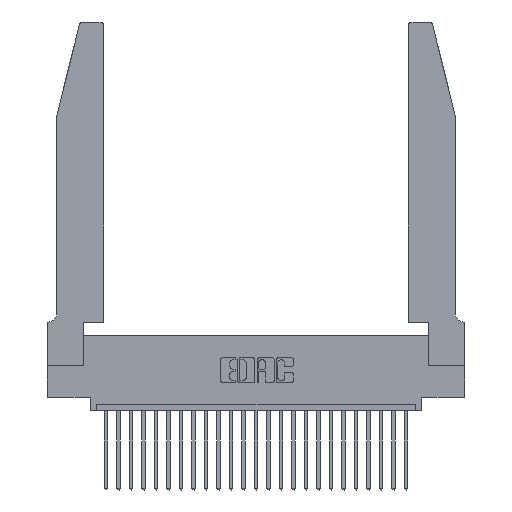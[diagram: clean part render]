
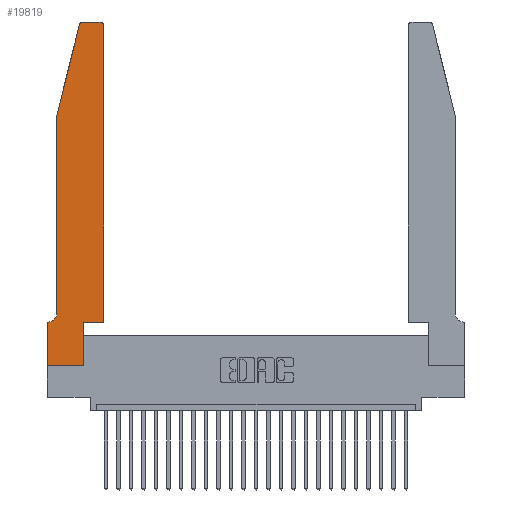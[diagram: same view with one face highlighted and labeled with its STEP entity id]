
A CAD part, top view. The second image highlights one B-rep face of the part: STEP entity #19819.
In plain terms, the highlighted planar face has unit normal (0, 0, 1).
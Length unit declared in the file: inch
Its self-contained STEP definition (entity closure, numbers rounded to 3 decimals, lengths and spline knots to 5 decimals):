
#22 = ORIENTED_EDGE ( 'NONE', *, *, #22327, .T. ) ;
#68 = VECTOR ( 'NONE', #6897, 39.37008 ) ;
#364 = CIRCLE ( 'NONE', #19131, 0.07 ) ;
#658 = LINE ( 'NONE', #8577, #12344 ) ;
#1362 = VERTEX_POINT ( 'NONE', #24633 ) ;
#1664 = ORIENTED_EDGE ( 'NONE', *, *, #7630, .T. ) ;
#1958 = VECTOR ( 'NONE', #2583, 39.37008 ) ;
#2416 = CARTESIAN_POINT ( 'NONE',  ( 0.0055, 0.35, 0.37 ) ) ;
#2583 = DIRECTION ( 'NONE',  ( 1., 0., 0. ) ) ;
#2667 = DIRECTION ( 'NONE',  ( 0., 1., 0. ) ) ;
#3139 = DIRECTION ( 'NONE',  ( 0., 1., 0. ) ) ;
#3328 = EDGE_CURVE ( 'NONE', #6459, #7437, #7722, .T. ) ;
#3610 = CARTESIAN_POINT ( 'NONE',  ( 0.284, 2.72, 0.37 ) ) ;
#4236 = LINE ( 'NONE', #19751, #19571 ) ;
#4491 = CARTESIAN_POINT ( 'NONE',  ( 0., 0., 0.37 ) ) ;
#5335 = EDGE_CURVE ( 'NONE', #22136, #1362, #6084, .T. ) ;
#5388 = ORIENTED_EDGE ( 'NONE', *, *, #3328, .T. ) ;
#5475 = DIRECTION ( 'NONE',  ( 0., -1., 0. ) ) ;
#5560 = EDGE_CURVE ( 'NONE', #18699, #16878, #7629, .T. ) ;
#5912 = CARTESIAN_POINT ( 'NONE',  ( 0.0755, 2., 0.37 ) ) ;
#6084 = LINE ( 'NONE', #16721, #68 ) ;
#6310 = CIRCLE ( 'NONE', #12311, 0.03 ) ;
#6459 = VERTEX_POINT ( 'NONE', #13502 ) ;
#6463 = CARTESIAN_POINT ( 'NONE',  ( 0., 0.35, 0.37 ) ) ;
#6897 = DIRECTION ( 'NONE',  ( -0.239, -0.971, 0. ) ) ;
#6904 = DIRECTION ( 'NONE',  ( 0., 0., 1. ) ) ;
#7437 = VERTEX_POINT ( 'NONE', #11404 ) ;
#7547 = EDGE_CURVE ( 'NONE', #16878, #6459, #9598, .T. ) ;
#7629 = LINE ( 'NONE', #8672, #1958 ) ;
#7630 = EDGE_CURVE ( 'NONE', #1362, #22819, #21156, .T. ) ;
#7655 = LINE ( 'NONE', #25362, #23326 ) ;
#7722 = LINE ( 'NONE', #12262, #18697 ) ;
#7840 = DIRECTION ( 'NONE',  ( 0., 0., 1. ) ) ;
#8106 = DIRECTION ( 'NONE',  ( -1., 0., 0. ) ) ;
#8119 = CARTESIAN_POINT ( 'NONE',  ( 0.2865, 0., 0.37 ) ) ;
#8397 = PLANE ( 'NONE',  #19398 ) ;
#8577 = CARTESIAN_POINT ( 'NONE',  ( 0.4505, 0.35, 0.37 ) ) ;
#8672 = CARTESIAN_POINT ( 'NONE',  ( 0., 0., 0.37 ) ) ;
#9000 = EDGE_CURVE ( 'NONE', #21776, #23937, #18585, .T. ) ;
#9338 = DIRECTION ( 'NONE',  ( 0., 0., -1. ) ) ;
#9598 = LINE ( 'NONE', #23118, #14314 ) ;
#9729 = CARTESIAN_POINT ( 'NONE',  ( 0.4205, 2.75, 0.37 ) ) ;
#10235 = DIRECTION ( 'NONE',  ( 1., 0., 0. ) ) ;
#10533 = ORIENTED_EDGE ( 'NONE', *, *, #5335, .T. ) ;
#11281 = ORIENTED_EDGE ( 'NONE', *, *, #12996, .T. ) ;
#11404 = CARTESIAN_POINT ( 'NONE',  ( 0.4505, 0.35, 0.37 ) ) ;
#11635 = ORIENTED_EDGE ( 'NONE', *, *, #17505, .T. ) ;
#12262 = CARTESIAN_POINT ( 'NONE',  ( 0.4505, 0.35, 0.37 ) ) ;
#12311 = AXIS2_PLACEMENT_3D ( 'NONE', #3610, #7840, #17645 ) ;
#12344 = VECTOR ( 'NONE', #2667, 39.37008 ) ;
#12996 = EDGE_CURVE ( 'NONE', #22819, #17789, #364, .T. ) ;
#13410 = DIRECTION ( 'NONE',  ( -1., 0., 0. ) ) ;
#13502 = CARTESIAN_POINT ( 'NONE',  ( 0.2865, 0.35, 0.37 ) ) ;
#13679 = VERTEX_POINT ( 'NONE', #23352 ) ;
#13755 = CARTESIAN_POINT ( 'NONE',  ( 0.284, 2.75, 0.37 ) ) ;
#14035 = VECTOR ( 'NONE', #8106, 39.37008 ) ;
#14158 = EDGE_CURVE ( 'NONE', #18980, #22136, #6310, .T. ) ;
#14314 = VECTOR ( 'NONE', #3139, 39.37008 ) ;
#14718 = ORIENTED_EDGE ( 'NONE', *, *, #7547, .T. ) ;
#14954 = ORIENTED_EDGE ( 'NONE', *, *, #24309, .T. ) ;
#16721 = CARTESIAN_POINT ( 'NONE',  ( 0.0755, 2., 0.37 ) ) ;
#16878 = VERTEX_POINT ( 'NONE', #8119 ) ;
#17505 = EDGE_CURVE ( 'NONE', #17789, #13679, #21199, .T. ) ;
#17555 = FACE_OUTER_BOUND ( 'NONE', #19304, .T. ) ;
#17645 = DIRECTION ( 'NONE',  ( 1., 0., 0. ) ) ;
#17789 = VERTEX_POINT ( 'NONE', #2416 ) ;
#18585 = CIRCLE ( 'NONE', #23219, 0.03 ) ;
#18697 = VECTOR ( 'NONE', #10235, 39.37008 ) ;
#18699 = VERTEX_POINT ( 'NONE', #4491 ) ;
#18793 = DIRECTION ( 'NONE',  ( 1., 0., 0. ) ) ;
#18980 = VERTEX_POINT ( 'NONE', #13755 ) ;
#19019 = DIRECTION ( 'NONE',  ( 0., 0., 1. ) ) ;
#19097 = DIRECTION ( 'NONE',  ( 1., 0., 0. ) ) ;
#19131 = AXIS2_PLACEMENT_3D ( 'NONE', #21377, #9338, #23485 ) ;
#19152 = CARTESIAN_POINT ( 'NONE',  ( 0.25487, 2.72718, 0.37 ) ) ;
#19304 = EDGE_LOOP ( 'NONE', ( #25159, #22742, #10533, #1664, #11281, #11635, #22, #25251, #14718, #5388, #14954, #23679 ) ) ;
#19398 = AXIS2_PLACEMENT_3D ( 'NONE', #6463, #6904, #18793 ) ;
#19571 = VECTOR ( 'NONE', #5475, 39.37008 ) ;
#19751 = CARTESIAN_POINT ( 'NONE',  ( 0., 0., 0.37 ) ) ;
#19819 = ADVANCED_FACE ( 'NONE', ( #17555 ), #8397, .T. ) ;
#19830 = DIRECTION ( 'NONE',  ( 0., -1., 0. ) ) ;
#21156 = LINE ( 'NONE', #5912, #24908 ) ;
#21199 = LINE ( 'NONE', #22874, #14035 ) ;
#21377 = CARTESIAN_POINT ( 'NONE',  ( 0.0055, 0.42, 0.37 ) ) ;
#21776 = VERTEX_POINT ( 'NONE', #21989 ) ;
#21854 = CARTESIAN_POINT ( 'NONE',  ( 0.0755, 0.42, 0.37 ) ) ;
#21989 = CARTESIAN_POINT ( 'NONE',  ( 0.4505, 2.72, 0.37 ) ) ;
#22136 = VERTEX_POINT ( 'NONE', #19152 ) ;
#22327 = EDGE_CURVE ( 'NONE', #13679, #18699, #4236, .T. ) ;
#22742 = ORIENTED_EDGE ( 'NONE', *, *, #14158, .T. ) ;
#22819 = VERTEX_POINT ( 'NONE', #21854 ) ;
#22874 = CARTESIAN_POINT ( 'NONE',  ( 0.0755, 0.35, 0.37 ) ) ;
#23118 = CARTESIAN_POINT ( 'NONE',  ( 0.2865, 0.35, 0.37 ) ) ;
#23219 = AXIS2_PLACEMENT_3D ( 'NONE', #23229, #19019, #19097 ) ;
#23229 = CARTESIAN_POINT ( 'NONE',  ( 0.4205, 2.72, 0.37 ) ) ;
#23326 = VECTOR ( 'NONE', #13410, 39.37008 ) ;
#23352 = CARTESIAN_POINT ( 'NONE',  ( 0., 0.35, 0.37 ) ) ;
#23485 = DIRECTION ( 'NONE',  ( -1., 0., 0. ) ) ;
#23679 = ORIENTED_EDGE ( 'NONE', *, *, #9000, .T. ) ;
#23917 = EDGE_CURVE ( 'NONE', #23937, #18980, #7655, .T. ) ;
#23937 = VERTEX_POINT ( 'NONE', #9729 ) ;
#24309 = EDGE_CURVE ( 'NONE', #7437, #21776, #658, .T. ) ;
#24633 = CARTESIAN_POINT ( 'NONE',  ( 0.0755, 2., 0.37 ) ) ;
#24908 = VECTOR ( 'NONE', #19830, 39.37008 ) ;
#25159 = ORIENTED_EDGE ( 'NONE', *, *, #23917, .T. ) ;
#25251 = ORIENTED_EDGE ( 'NONE', *, *, #5560, .T. ) ;
#25362 = CARTESIAN_POINT ( 'NONE',  ( 0.2605, 2.75, 0.37 ) ) ;
